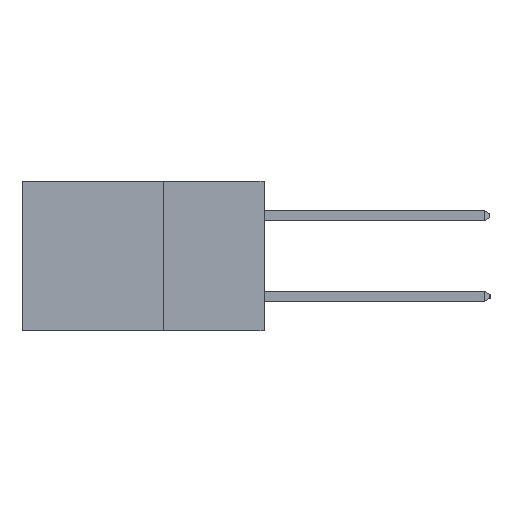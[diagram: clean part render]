
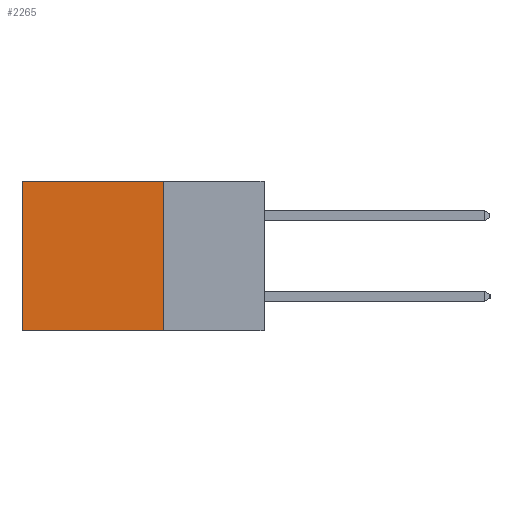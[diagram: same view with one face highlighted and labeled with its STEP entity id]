
A CAD part, left-side view. The second image highlights one B-rep face of the part: STEP entity #2265.
In plain terms, the highlighted planar face has unit normal (-1, 0, 0).
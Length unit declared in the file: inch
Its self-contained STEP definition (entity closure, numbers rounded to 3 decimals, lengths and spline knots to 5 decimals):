
#131 = ORIENTED_EDGE ( 'NONE', *, *, #2193, .T. ) ;
#2193 = EDGE_CURVE ( 'NONE', #6159, #6797, #22135, .T. ) ;
#2265 = ADVANCED_FACE ( 'NONE', ( #20363 ), #13705, .F. ) ;
#2624 = VECTOR ( 'NONE', #22288, 39.37008 ) ;
#4185 = VECTOR ( 'NONE', #21472, 39.37008 ) ;
#4915 = CARTESIAN_POINT ( 'NONE',  ( 0.2615, 0.25, -0.37 ) ) ;
#5034 = CARTESIAN_POINT ( 'NONE',  ( 0.2615, 0.25, 0. ) ) ;
#5483 = CARTESIAN_POINT ( 'NONE',  ( 0.2615, 0.6, 0. ) ) ;
#6159 = VERTEX_POINT ( 'NONE', #5483 ) ;
#6680 = EDGE_CURVE ( 'NONE', #20115, #6159, #10349, .T. ) ;
#6797 = VERTEX_POINT ( 'NONE', #15079 ) ;
#6932 = DIRECTION ( 'NONE',  ( 0., 1., 0. ) ) ;
#8042 = CARTESIAN_POINT ( 'NONE',  ( 0.2615, 0.25, -0.37 ) ) ;
#10349 = LINE ( 'NONE', #24170, #19928 ) ;
#12001 = AXIS2_PLACEMENT_3D ( 'NONE', #13516, #13294, #12568 ) ;
#12568 = DIRECTION ( 'NONE',  ( 0., 0., -1. ) ) ;
#13044 = LINE ( 'NONE', #4915, #2624 ) ;
#13203 = VECTOR ( 'NONE', #16967, 39.37008 ) ;
#13294 = DIRECTION ( 'NONE',  ( 1., 0., 0. ) ) ;
#13516 = CARTESIAN_POINT ( 'NONE',  ( 0.2615, 0.25, -0.37 ) ) ;
#13705 = PLANE ( 'NONE',  #12001 ) ;
#15079 = CARTESIAN_POINT ( 'NONE',  ( 0.2615, 0.6, -0.37 ) ) ;
#15172 = LINE ( 'NONE', #8042, #4185 ) ;
#15724 = ORIENTED_EDGE ( 'NONE', *, *, #6680, .T. ) ;
#16546 = EDGE_LOOP ( 'NONE', ( #131, #21813, #21135, #15724 ) ) ;
#16967 = DIRECTION ( 'NONE',  ( 0., 0., -1. ) ) ;
#17146 = CARTESIAN_POINT ( 'NONE',  ( 0.2615, 0.6, -0.37 ) ) ;
#18405 = VERTEX_POINT ( 'NONE', #23519 ) ;
#19928 = VECTOR ( 'NONE', #6932, 39.37008 ) ;
#20115 = VERTEX_POINT ( 'NONE', #5034 ) ;
#20363 = FACE_OUTER_BOUND ( 'NONE', #16546, .T. ) ;
#21135 = ORIENTED_EDGE ( 'NONE', *, *, #22203, .F. ) ;
#21472 = DIRECTION ( 'NONE',  ( 0., 0., -1. ) ) ;
#21813 = ORIENTED_EDGE ( 'NONE', *, *, #22505, .F. ) ;
#22135 = LINE ( 'NONE', #17146, #13203 ) ;
#22203 = EDGE_CURVE ( 'NONE', #20115, #18405, #15172, .T. ) ;
#22288 = DIRECTION ( 'NONE',  ( 0., 1., 0. ) ) ;
#22505 = EDGE_CURVE ( 'NONE', #18405, #6797, #13044, .T. ) ;
#23519 = CARTESIAN_POINT ( 'NONE',  ( 0.2615, 0.25, -0.37 ) ) ;
#24170 = CARTESIAN_POINT ( 'NONE',  ( 0.2615, 0.25, 0. ) ) ;
